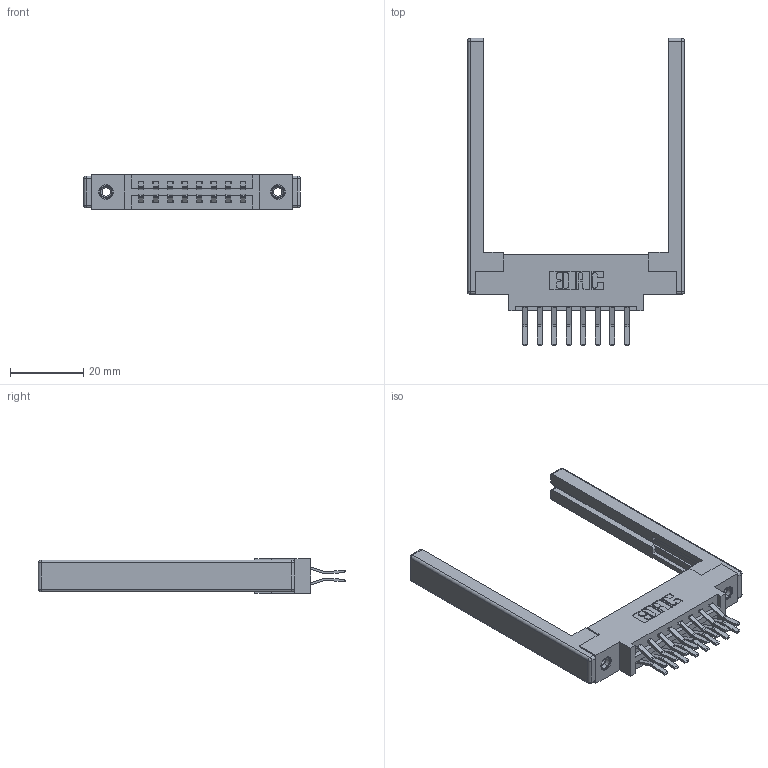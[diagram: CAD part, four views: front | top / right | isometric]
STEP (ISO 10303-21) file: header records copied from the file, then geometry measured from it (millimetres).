
FILE_DESCRIPTION (( 'STEP AP203' ), '1' );
FILE_NAME ('387-016-560-868.STEP', '2019-10-16T00:21:30', ( '' ), ( '' ), 'SwSTEP 2.0', 'SolidWorks 2016', '' );
FILE_SCHEMA (( 'CONFIG_CONTROL_DESIGN' ));
Length unit declared in the file: inch
Products named in the file (5): 345-250-001_345-250-001-102; 307-220-068; 345-292-001_560 Tail; 387-016-560-868; 337 Part_0.170 Offset - 0.156 Dia-TI
Assembly tree (21 placements, depth 2):
  387-016-560-868
    337 Part_0.170 Offset - 0.156 Dia-TI
    345-292-001_560 Tail  x16
    345-250-001_345-250-001-102  x2
    307-220-068  x2
Bounding box: 59.13 x 83.84 x 9.4 mm (x, y, z)
Volume: 10151.3 mm3; surface area: 10634.5 mm2
Topology: 21 solids, 21 shells, 1168 faces, 3385 edges, 2214 vertices
Faces by surface type: plane 770, cylinder 374, cone 12, sphere 8, torus 4
Entity records: 13580 total; most frequent: CARTESIAN_POINT 2283, ORIENTED_EDGE 2208, DIRECTION 2078, EDGE_CURVE 1104, VECTOR 922, LINE 922, VERTEX_POINT 726, AXIS2_PLACEMENT_3D 578
